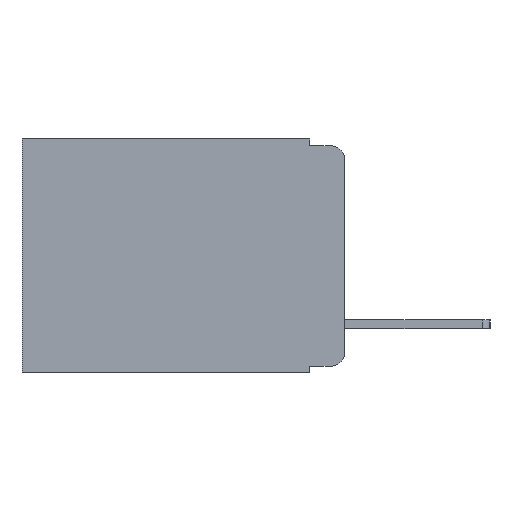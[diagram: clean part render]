
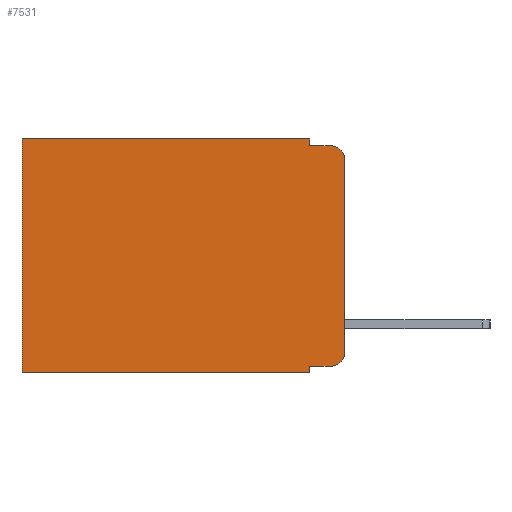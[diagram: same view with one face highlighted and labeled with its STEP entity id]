
A CAD part, left-side view. The second image highlights one B-rep face of the part: STEP entity #7531.
In plain terms, the highlighted planar face has unit normal (-1, 0, 0).
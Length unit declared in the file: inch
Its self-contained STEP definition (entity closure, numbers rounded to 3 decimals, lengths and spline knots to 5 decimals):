
#157 = LINE ( 'NONE', #413, #9951 ) ;
#340 = ORIENTED_EDGE ( 'NONE', *, *, #1664, .T. ) ;
#411 = CARTESIAN_POINT ( 'NONE',  ( 0.298, 0., 0. ) ) ;
#413 = CARTESIAN_POINT ( 'NONE',  ( 0.298, 0.473, 0. ) ) ;
#1030 = ORIENTED_EDGE ( 'NONE', *, *, #8422, .F. ) ;
#1480 = LINE ( 'NONE', #2968, #6666 ) ;
#1664 = EDGE_CURVE ( 'NONE', #4492, #8802, #4806, .T. ) ;
#1754 = CARTESIAN_POINT ( 'NONE',  ( 0.298, 0.02, -0.333 ) ) ;
#1816 = ORIENTED_EDGE ( 'NONE', *, *, #11804, .F. ) ;
#2556 = EDGE_CURVE ( 'NONE', #13296, #3917, #10913, .T. ) ;
#2643 = VERTEX_POINT ( 'NONE', #13071 ) ;
#2659 = VECTOR ( 'NONE', #8979, 39.37008 ) ;
#2848 = DIRECTION ( 'NONE',  ( 0., 1., 0. ) ) ;
#2952 = EDGE_CURVE ( 'NONE', #13296, #3947, #2974, .T. ) ;
#2968 = CARTESIAN_POINT ( 'NONE',  ( 0.298, 0.051, -0.01 ) ) ;
#2974 = LINE ( 'NONE', #12608, #2659 ) ;
#3033 = VERTEX_POINT ( 'NONE', #3515 ) ;
#3407 = CIRCLE ( 'NONE', #9145, 0.02 ) ;
#3413 = ORIENTED_EDGE ( 'NONE', *, *, #2556, .T. ) ;
#3464 = ORIENTED_EDGE ( 'NONE', *, *, #11483, .T. ) ;
#3515 = CARTESIAN_POINT ( 'NONE',  ( 0.298, 0.02, -0.01 ) ) ;
#3597 = DIRECTION ( 'NONE',  ( 0., 0., -1. ) ) ;
#3664 = ORIENTED_EDGE ( 'NONE', *, *, #7631, .F. ) ;
#3917 = VERTEX_POINT ( 'NONE', #9351 ) ;
#3947 = VERTEX_POINT ( 'NONE', #5035 ) ;
#4145 = ORIENTED_EDGE ( 'NONE', *, *, #13026, .F. ) ;
#4280 = CARTESIAN_POINT ( 'NONE',  ( 0.298, 0.051, 0. ) ) ;
#4492 = VERTEX_POINT ( 'NONE', #10299 ) ;
#4575 = FACE_OUTER_BOUND ( 'NONE', #5970, .T. ) ;
#4640 = VECTOR ( 'NONE', #10714, 39.37008 ) ;
#4806 = LINE ( 'NONE', #5586, #9994 ) ;
#4811 = DIRECTION ( 'NONE',  ( 0., 0., -1. ) ) ;
#4870 = EDGE_CURVE ( 'NONE', #2643, #3033, #3407, .T. ) ;
#4885 = DIRECTION ( 'NONE',  ( 0., -1., 0. ) ) ;
#4949 = ORIENTED_EDGE ( 'NONE', *, *, #6859, .T. ) ;
#4966 = LINE ( 'NONE', #12725, #4640 ) ;
#5035 = CARTESIAN_POINT ( 'NONE',  ( 0.298, 0.051, -0.01 ) ) ;
#5203 = VERTEX_POINT ( 'NONE', #9418 ) ;
#5586 = CARTESIAN_POINT ( 'NONE',  ( 0.298, 0.051, -0.333 ) ) ;
#5854 = DIRECTION ( 'NONE',  ( 0., 1., 0. ) ) ;
#5858 = ORIENTED_EDGE ( 'NONE', *, *, #2952, .F. ) ;
#5970 = EDGE_LOOP ( 'NONE', ( #1816, #6706, #1030, #5858, #3413, #4949, #4145, #3664, #340, #3464 ) ) ;
#6055 = CARTESIAN_POINT ( 'NONE',  ( 0.298, 0.051, -0.343 ) ) ;
#6066 = DIRECTION ( 'NONE',  ( -1., 0., 0. ) ) ;
#6094 = DIRECTION ( 'NONE',  ( 0., -1., 0. ) ) ;
#6176 = VERTEX_POINT ( 'NONE', #6055 ) ;
#6666 = VECTOR ( 'NONE', #6094, 39.37008 ) ;
#6706 = ORIENTED_EDGE ( 'NONE', *, *, #4870, .T. ) ;
#6721 = DIRECTION ( 'NONE',  ( 0., 0., -1. ) ) ;
#6850 = CARTESIAN_POINT ( 'NONE',  ( 0.298, 0.051, 0. ) ) ;
#6859 = EDGE_CURVE ( 'NONE', #3917, #5203, #157, .T. ) ;
#7531 = ADVANCED_FACE ( 'NONE', ( #4575 ), #11824, .F. ) ;
#7583 = DIRECTION ( 'NONE',  ( -1., 0., 0. ) ) ;
#7631 = EDGE_CURVE ( 'NONE', #4492, #6176, #9107, .T. ) ;
#7718 = CARTESIAN_POINT ( 'NONE',  ( 0.298, 0., 0. ) ) ;
#7863 = VECTOR ( 'NONE', #5854, 39.37008 ) ;
#8422 = EDGE_CURVE ( 'NONE', #3947, #3033, #1480, .T. ) ;
#8451 = VECTOR ( 'NONE', #4811, 39.37008 ) ;
#8802 = VERTEX_POINT ( 'NONE', #1754 ) ;
#8979 = DIRECTION ( 'NONE',  ( 0., 0., -1. ) ) ;
#9107 = LINE ( 'NONE', #6850, #8451 ) ;
#9145 = AXIS2_PLACEMENT_3D ( 'NONE', #9929, #7583, #13178 ) ;
#9179 = CIRCLE ( 'NONE', #12928, 0.02 ) ;
#9351 = CARTESIAN_POINT ( 'NONE',  ( 0.298, 0.473, 0. ) ) ;
#9418 = CARTESIAN_POINT ( 'NONE',  ( 0.298, 0.473, -0.343 ) ) ;
#9869 = LINE ( 'NONE', #12132, #12567 ) ;
#9929 = CARTESIAN_POINT ( 'NONE',  ( 0.298, 0.02, -0.03 ) ) ;
#9951 = VECTOR ( 'NONE', #3597, 39.37008 ) ;
#9994 = VECTOR ( 'NONE', #4885, 39.37008 ) ;
#10299 = CARTESIAN_POINT ( 'NONE',  ( 0.298, 0.051, -0.333 ) ) ;
#10714 = DIRECTION ( 'NONE',  ( 0., 0., -1. ) ) ;
#10913 = LINE ( 'NONE', #411, #7863 ) ;
#11001 = AXIS2_PLACEMENT_3D ( 'NONE', #7718, #12872, #6721 ) ;
#11314 = VERTEX_POINT ( 'NONE', #12930 ) ;
#11483 = EDGE_CURVE ( 'NONE', #8802, #11314, #9179, .T. ) ;
#11804 = EDGE_CURVE ( 'NONE', #2643, #11314, #4966, .T. ) ;
#11824 = PLANE ( 'NONE',  #11001 ) ;
#12132 = CARTESIAN_POINT ( 'NONE',  ( 0.298, 0., -0.343 ) ) ;
#12235 = CARTESIAN_POINT ( 'NONE',  ( 0.298, 0.02, -0.313 ) ) ;
#12567 = VECTOR ( 'NONE', #2848, 39.37008 ) ;
#12608 = CARTESIAN_POINT ( 'NONE',  ( 0.298, 0.051, 0. ) ) ;
#12725 = CARTESIAN_POINT ( 'NONE',  ( 0.298, 0., 0. ) ) ;
#12872 = DIRECTION ( 'NONE',  ( 1., 0., 0. ) ) ;
#12928 = AXIS2_PLACEMENT_3D ( 'NONE', #12235, #6066, #13270 ) ;
#12930 = CARTESIAN_POINT ( 'NONE',  ( 0.298, 0., -0.313 ) ) ;
#13026 = EDGE_CURVE ( 'NONE', #6176, #5203, #9869, .T. ) ;
#13071 = CARTESIAN_POINT ( 'NONE',  ( 0.298, 0., -0.03 ) ) ;
#13178 = DIRECTION ( 'NONE',  ( 0., 0., -1. ) ) ;
#13270 = DIRECTION ( 'NONE',  ( 0., 0., -1. ) ) ;
#13296 = VERTEX_POINT ( 'NONE', #4280 ) ;
